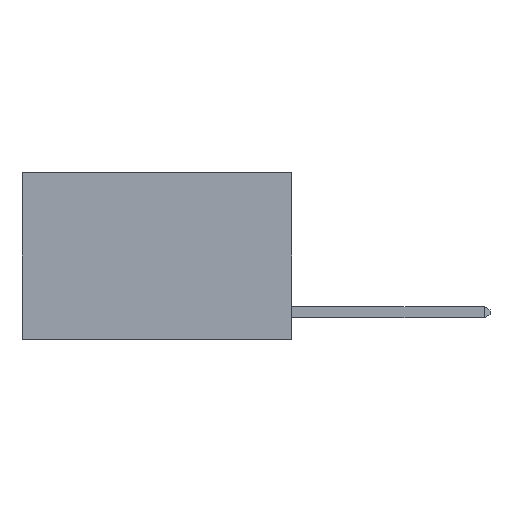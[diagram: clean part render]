
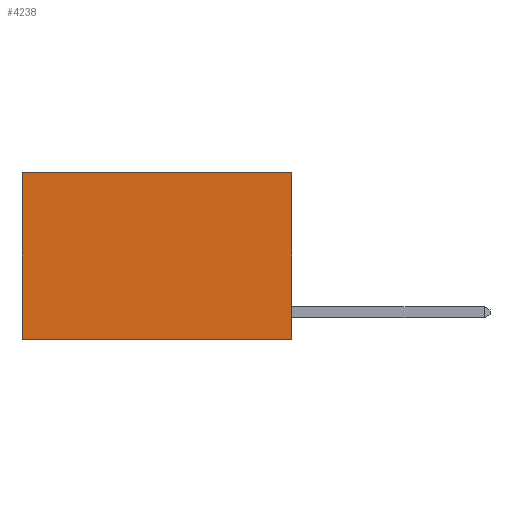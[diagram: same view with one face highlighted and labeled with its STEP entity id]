
A CAD part, left-side view. The second image highlights one B-rep face of the part: STEP entity #4238.
In plain terms, the highlighted planar face has unit normal (-1, 0, 0).
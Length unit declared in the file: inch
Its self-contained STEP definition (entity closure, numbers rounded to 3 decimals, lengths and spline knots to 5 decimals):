
#115 = LINE ( 'NONE', #7405, #8986 ) ;
#181 = DIRECTION ( 'NONE',  ( 0., 0., -1. ) ) ;
#283 = PLANE ( 'NONE',  #1699 ) ;
#577 = ORIENTED_EDGE ( 'NONE', *, *, #4141, .T. ) ;
#743 = ORIENTED_EDGE ( 'NONE', *, *, #1183, .F. ) ;
#876 = CARTESIAN_POINT ( 'NONE',  ( 0.2625, 0., 0. ) ) ;
#1162 = CARTESIAN_POINT ( 'NONE',  ( 0.2625, 0., 0. ) ) ;
#1183 = EDGE_CURVE ( 'NONE', #7580, #2224, #7882, .T. ) ;
#1699 = AXIS2_PLACEMENT_3D ( 'NONE', #1735, #6826, #2465 ) ;
#1735 = CARTESIAN_POINT ( 'NONE',  ( 0.2625, 0., 0. ) ) ;
#2001 = CARTESIAN_POINT ( 'NONE',  ( 0.2625, 0., -0.37 ) ) ;
#2044 = VERTEX_POINT ( 'NONE', #7059 ) ;
#2224 = VERTEX_POINT ( 'NONE', #8060 ) ;
#2240 = VECTOR ( 'NONE', #3754, 39.37008 ) ;
#2465 = DIRECTION ( 'NONE',  ( 0., 0., -1. ) ) ;
#2929 = EDGE_CURVE ( 'NONE', #2966, #2044, #115, .T. ) ;
#2966 = VERTEX_POINT ( 'NONE', #8752 ) ;
#3019 = LINE ( 'NONE', #2001, #6684 ) ;
#3193 = ORIENTED_EDGE ( 'NONE', *, *, #3909, .F. ) ;
#3754 = DIRECTION ( 'NONE',  ( 0., 1., 0. ) ) ;
#3909 = EDGE_CURVE ( 'NONE', #2224, #2044, #3019, .T. ) ;
#3921 = ORIENTED_EDGE ( 'NONE', *, *, #2929, .T. ) ;
#3999 = VECTOR ( 'NONE', #5721, 39.37008 ) ;
#4141 = EDGE_CURVE ( 'NONE', #7580, #2966, #6112, .T. ) ;
#4238 = ADVANCED_FACE ( 'NONE', ( #7127 ), #283, .F. ) ;
#5721 = DIRECTION ( 'NONE',  ( 0., 0., -1. ) ) ;
#6112 = LINE ( 'NONE', #876, #2240 ) ;
#6359 = DIRECTION ( 'NONE',  ( 0., 1., 0. ) ) ;
#6617 = EDGE_LOOP ( 'NONE', ( #3921, #3193, #743, #577 ) ) ;
#6684 = VECTOR ( 'NONE', #6359, 39.37008 ) ;
#6826 = DIRECTION ( 'NONE',  ( 1., 0., 0. ) ) ;
#7059 = CARTESIAN_POINT ( 'NONE',  ( 0.2625, 0.6, -0.37 ) ) ;
#7127 = FACE_OUTER_BOUND ( 'NONE', #6617, .T. ) ;
#7306 = CARTESIAN_POINT ( 'NONE',  ( 0.2625, 0., 0. ) ) ;
#7405 = CARTESIAN_POINT ( 'NONE',  ( 0.2625, 0.6, 0. ) ) ;
#7580 = VERTEX_POINT ( 'NONE', #1162 ) ;
#7882 = LINE ( 'NONE', #7306, #3999 ) ;
#8060 = CARTESIAN_POINT ( 'NONE',  ( 0.2625, 0., -0.37 ) ) ;
#8752 = CARTESIAN_POINT ( 'NONE',  ( 0.2625, 0.6, 0. ) ) ;
#8986 = VECTOR ( 'NONE', #181, 39.37008 ) ;
